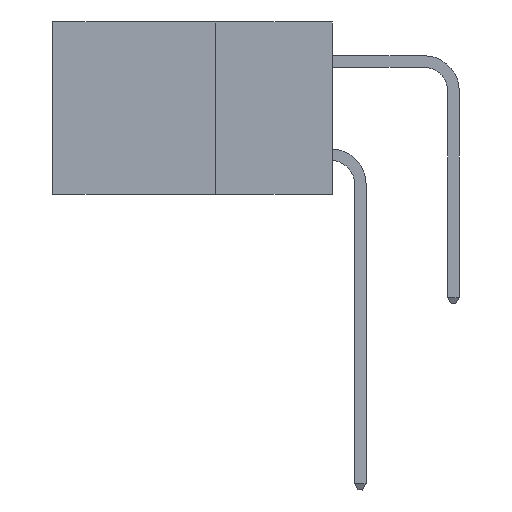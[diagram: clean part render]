
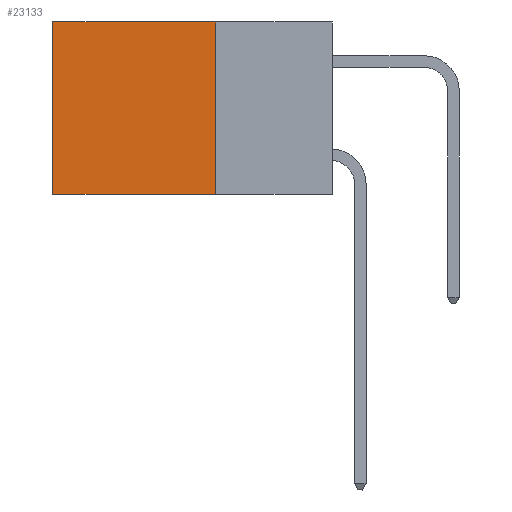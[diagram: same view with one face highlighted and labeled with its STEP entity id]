
A CAD part, left-side view. The second image highlights one B-rep face of the part: STEP entity #23133.
In plain terms, the highlighted planar face has unit normal (-1, 0, 0).
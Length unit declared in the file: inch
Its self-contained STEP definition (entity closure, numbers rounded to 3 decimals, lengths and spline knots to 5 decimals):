
#2620 = VECTOR ( 'NONE', #4739, 39.37008 ) ;
#2702 = DIRECTION ( 'NONE',  ( 0., 1., 0. ) ) ;
#2813 = ORIENTED_EDGE ( 'NONE', *, *, #4032, .F. ) ;
#3078 = VECTOR ( 'NONE', #24686, 39.37008 ) ;
#3483 = CARTESIAN_POINT ( 'NONE',  ( 0.2615, 0.6, -0.37 ) ) ;
#3520 = EDGE_CURVE ( 'NONE', #18503, #19358, #19768, .T. ) ;
#3624 = ORIENTED_EDGE ( 'NONE', *, *, #3520, .T. ) ;
#4032 = EDGE_CURVE ( 'NONE', #15950, #19358, #24305, .T. ) ;
#4739 = DIRECTION ( 'NONE',  ( 0., 0., -1. ) ) ;
#5736 = DIRECTION ( 'NONE',  ( 0., 0., -1. ) ) ;
#6148 = EDGE_CURVE ( 'NONE', #10420, #15950, #20493, .T. ) ;
#6469 = EDGE_CURVE ( 'NONE', #10420, #18503, #11955, .T. ) ;
#7479 = CARTESIAN_POINT ( 'NONE',  ( 0.2615, 0.25, -0.37 ) ) ;
#8004 = CARTESIAN_POINT ( 'NONE',  ( 0.2615, 0.25, -0.37 ) ) ;
#8346 = VECTOR ( 'NONE', #12715, 39.37008 ) ;
#9770 = AXIS2_PLACEMENT_3D ( 'NONE', #7479, #20887, #5736 ) ;
#10420 = VERTEX_POINT ( 'NONE', #10908 ) ;
#10589 = CARTESIAN_POINT ( 'NONE',  ( 0.2615, 0.25, -0.37 ) ) ;
#10908 = CARTESIAN_POINT ( 'NONE',  ( 0.2615, 0.25, 0. ) ) ;
#11955 = LINE ( 'NONE', #17866, #13162 ) ;
#12715 = DIRECTION ( 'NONE',  ( 0., 0., -1. ) ) ;
#13162 = VECTOR ( 'NONE', #2702, 39.37008 ) ;
#15950 = VERTEX_POINT ( 'NONE', #8004 ) ;
#17866 = CARTESIAN_POINT ( 'NONE',  ( 0.2615, 0.25, 0. ) ) ;
#18503 = VERTEX_POINT ( 'NONE', #19928 ) ;
#18863 = EDGE_LOOP ( 'NONE', ( #3624, #2813, #19608, #22298 ) ) ;
#19358 = VERTEX_POINT ( 'NONE', #3483 ) ;
#19608 = ORIENTED_EDGE ( 'NONE', *, *, #6148, .F. ) ;
#19768 = LINE ( 'NONE', #21893, #2620 ) ;
#19928 = CARTESIAN_POINT ( 'NONE',  ( 0.2615, 0.6, 0. ) ) ;
#20493 = LINE ( 'NONE', #10589, #8346 ) ;
#20887 = DIRECTION ( 'NONE',  ( 1., 0., 0. ) ) ;
#20934 = CARTESIAN_POINT ( 'NONE',  ( 0.2615, 0.25, -0.37 ) ) ;
#21893 = CARTESIAN_POINT ( 'NONE',  ( 0.2615, 0.6, -0.37 ) ) ;
#22298 = ORIENTED_EDGE ( 'NONE', *, *, #6469, .T. ) ;
#23014 = FACE_OUTER_BOUND ( 'NONE', #18863, .T. ) ;
#23133 = ADVANCED_FACE ( 'NONE', ( #23014 ), #24509, .F. ) ;
#24305 = LINE ( 'NONE', #20934, #3078 ) ;
#24509 = PLANE ( 'NONE',  #9770 ) ;
#24686 = DIRECTION ( 'NONE',  ( 0., 1., 0. ) ) ;
